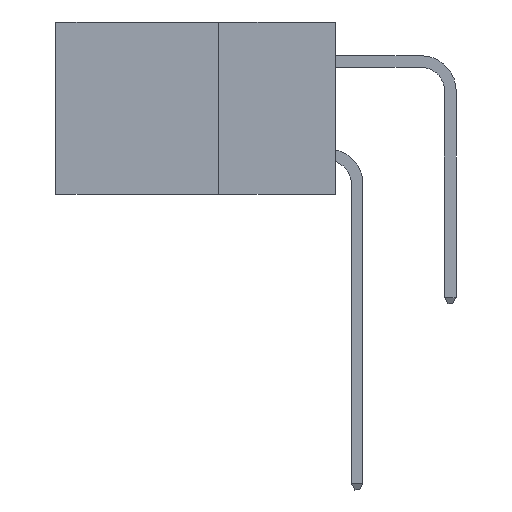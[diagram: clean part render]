
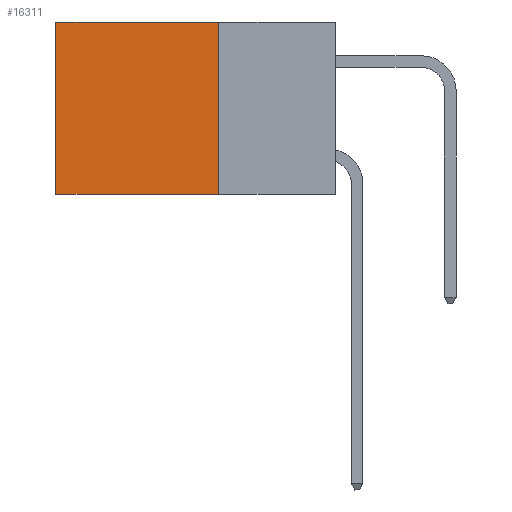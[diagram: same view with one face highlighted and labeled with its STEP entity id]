
A CAD part, left-side view. The second image highlights one B-rep face of the part: STEP entity #16311.
In plain terms, the highlighted planar face has unit normal (-1, 0, 0).
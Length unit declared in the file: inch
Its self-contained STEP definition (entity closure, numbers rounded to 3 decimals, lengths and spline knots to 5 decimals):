
#2246 = DIRECTION ( 'NONE',  ( 0., 0., -1. ) ) ;
#2864 = ORIENTED_EDGE ( 'NONE', *, *, #17106, .F. ) ;
#3938 = CARTESIAN_POINT ( 'NONE',  ( 0.2875, 0.25, -0.37 ) ) ;
#4218 = ORIENTED_EDGE ( 'NONE', *, *, #13384, .F. ) ;
#4829 = FACE_OUTER_BOUND ( 'NONE', #8915, .T. ) ;
#5257 = EDGE_CURVE ( 'NONE', #8441, #18656, #9934, .T. ) ;
#5869 = ORIENTED_EDGE ( 'NONE', *, *, #5257, .T. ) ;
#5897 = DIRECTION ( 'NONE',  ( 0., 1., 0. ) ) ;
#5974 = VECTOR ( 'NONE', #20027, 39.37008 ) ;
#6571 = LINE ( 'NONE', #18228, #5974 ) ;
#6581 = VECTOR ( 'NONE', #2246, 39.37008 ) ;
#7296 = ORIENTED_EDGE ( 'NONE', *, *, #19631, .T. ) ;
#7333 = VERTEX_POINT ( 'NONE', #21254 ) ;
#8441 = VERTEX_POINT ( 'NONE', #22461 ) ;
#8915 = EDGE_LOOP ( 'NONE', ( #7296, #4218, #2864, #5869 ) ) ;
#9345 = VECTOR ( 'NONE', #14253, 39.37008 ) ;
#9934 = LINE ( 'NONE', #12420, #9345 ) ;
#9979 = CARTESIAN_POINT ( 'NONE',  ( 0.2875, 0.6, 0. ) ) ;
#10473 = DIRECTION ( 'NONE',  ( 0., 0., -1. ) ) ;
#12074 = VECTOR ( 'NONE', #5897, 39.37008 ) ;
#12420 = CARTESIAN_POINT ( 'NONE',  ( 0.2875, 0.25, 0. ) ) ;
#13384 = EDGE_CURVE ( 'NONE', #15424, #7333, #17521, .T. ) ;
#14253 = DIRECTION ( 'NONE',  ( 0., 1., 0. ) ) ;
#15424 = VERTEX_POINT ( 'NONE', #17436 ) ;
#15493 = CARTESIAN_POINT ( 'NONE',  ( 0.2875, 0.6, 0. ) ) ;
#15902 = LINE ( 'NONE', #9979, #6581 ) ;
#15922 = CARTESIAN_POINT ( 'NONE',  ( 0.2875, 0.25, 0. ) ) ;
#16311 = ADVANCED_FACE ( 'NONE', ( #4829 ), #19597, .F. ) ;
#17106 = EDGE_CURVE ( 'NONE', #8441, #15424, #6571, .T. ) ;
#17436 = CARTESIAN_POINT ( 'NONE',  ( 0.2875, 0.25, -0.37 ) ) ;
#17521 = LINE ( 'NONE', #3938, #12074 ) ;
#18228 = CARTESIAN_POINT ( 'NONE',  ( 0.2875, 0.25, 0. ) ) ;
#18656 = VERTEX_POINT ( 'NONE', #15493 ) ;
#19597 = PLANE ( 'NONE',  #21510 ) ;
#19631 = EDGE_CURVE ( 'NONE', #18656, #7333, #15902, .T. ) ;
#20027 = DIRECTION ( 'NONE',  ( 0., 0., -1. ) ) ;
#21254 = CARTESIAN_POINT ( 'NONE',  ( 0.2875, 0.6, -0.37 ) ) ;
#21387 = DIRECTION ( 'NONE',  ( 1., 0., 0. ) ) ;
#21510 = AXIS2_PLACEMENT_3D ( 'NONE', #15922, #21387, #10473 ) ;
#22461 = CARTESIAN_POINT ( 'NONE',  ( 0.2875, 0.25, 0. ) ) ;
